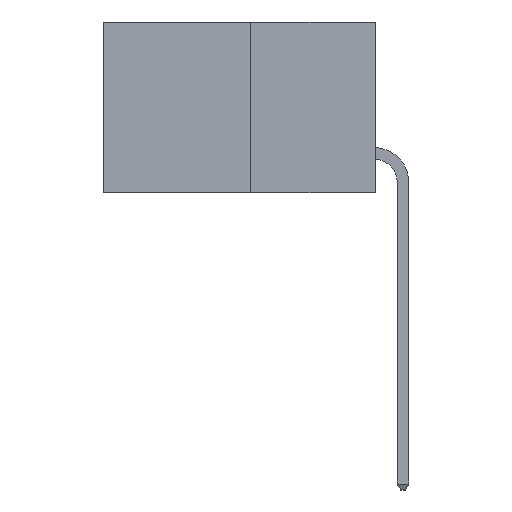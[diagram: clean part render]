
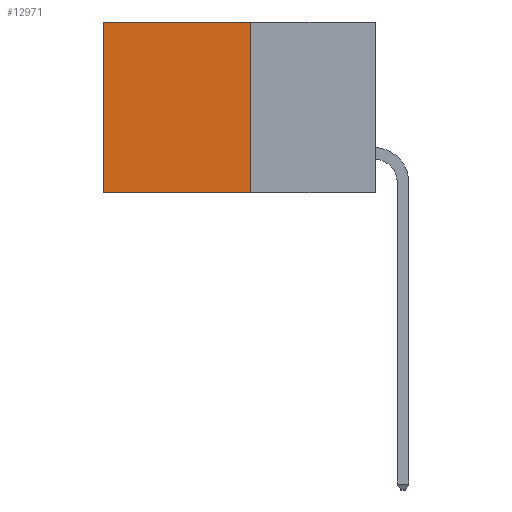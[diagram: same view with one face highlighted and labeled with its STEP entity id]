
A CAD part, left-side view. The second image highlights one B-rep face of the part: STEP entity #12971.
In plain terms, the highlighted planar face has unit normal (-1, 0, 0).
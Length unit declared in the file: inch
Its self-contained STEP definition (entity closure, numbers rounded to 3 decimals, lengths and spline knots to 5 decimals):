
#679 = ORIENTED_EDGE ( 'NONE', *, *, #19320, .F. ) ;
#828 = EDGE_LOOP ( 'NONE', ( #5585, #19773, #679, #19177 ) ) ;
#1025 = VECTOR ( 'NONE', #3351, 39.37008 ) ;
#1977 = DIRECTION ( 'NONE',  ( 0., 1., 0. ) ) ;
#3108 = PLANE ( 'NONE',  #26137 ) ;
#3351 = DIRECTION ( 'NONE',  ( 0., 0., -1. ) ) ;
#4343 = VERTEX_POINT ( 'NONE', #24221 ) ;
#5585 = ORIENTED_EDGE ( 'NONE', *, *, #10947, .T. ) ;
#5764 = DIRECTION ( 'NONE',  ( 0., 0., -1. ) ) ;
#6153 = LINE ( 'NONE', #9935, #31512 ) ;
#7719 = VECTOR ( 'NONE', #32281, 39.37008 ) ;
#9935 = CARTESIAN_POINT ( 'NONE',  ( 0.277, 0.27, -0.37 ) ) ;
#10947 = EDGE_CURVE ( 'NONE', #22479, #16292, #28228, .T. ) ;
#12176 = CARTESIAN_POINT ( 'NONE',  ( 0.277, 0.27, 0. ) ) ;
#12971 = ADVANCED_FACE ( 'NONE', ( #31982 ), #3108, .F. ) ;
#13678 = CARTESIAN_POINT ( 'NONE',  ( 0.277, 0.59, -0.37 ) ) ;
#15442 = DIRECTION ( 'NONE',  ( 0., 0., -1. ) ) ;
#15594 = EDGE_CURVE ( 'NONE', #4343, #22479, #28666, .T. ) ;
#15969 = CARTESIAN_POINT ( 'NONE',  ( 0.277, 0.27, -0.37 ) ) ;
#16292 = VERTEX_POINT ( 'NONE', #29968 ) ;
#16571 = CARTESIAN_POINT ( 'NONE',  ( 0.277, 0.59, 0. ) ) ;
#17004 = VERTEX_POINT ( 'NONE', #24062 ) ;
#19177 = ORIENTED_EDGE ( 'NONE', *, *, #15594, .T. ) ;
#19254 = LINE ( 'NONE', #32990, #25146 ) ;
#19320 = EDGE_CURVE ( 'NONE', #4343, #17004, #19254, .T. ) ;
#19773 = ORIENTED_EDGE ( 'NONE', *, *, #27834, .F. ) ;
#21062 = DIRECTION ( 'NONE',  ( 1., 0., 0. ) ) ;
#22479 = VERTEX_POINT ( 'NONE', #16571 ) ;
#24062 = CARTESIAN_POINT ( 'NONE',  ( 0.277, 0.27, -0.37 ) ) ;
#24221 = CARTESIAN_POINT ( 'NONE',  ( 0.277, 0.27, 0. ) ) ;
#25146 = VECTOR ( 'NONE', #15442, 39.37008 ) ;
#26137 = AXIS2_PLACEMENT_3D ( 'NONE', #15969, #21062, #5764 ) ;
#27834 = EDGE_CURVE ( 'NONE', #17004, #16292, #6153, .T. ) ;
#28228 = LINE ( 'NONE', #13678, #1025 ) ;
#28666 = LINE ( 'NONE', #12176, #7719 ) ;
#29968 = CARTESIAN_POINT ( 'NONE',  ( 0.277, 0.59, -0.37 ) ) ;
#31512 = VECTOR ( 'NONE', #1977, 39.37008 ) ;
#31982 = FACE_OUTER_BOUND ( 'NONE', #828, .T. ) ;
#32281 = DIRECTION ( 'NONE',  ( 0., 1., 0. ) ) ;
#32990 = CARTESIAN_POINT ( 'NONE',  ( 0.277, 0.27, -0.37 ) ) ;
